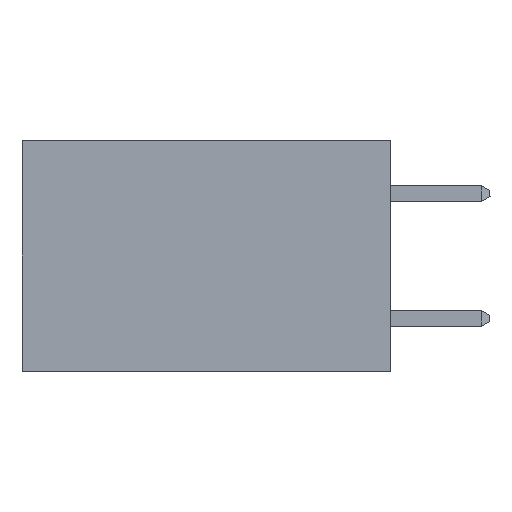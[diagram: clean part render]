
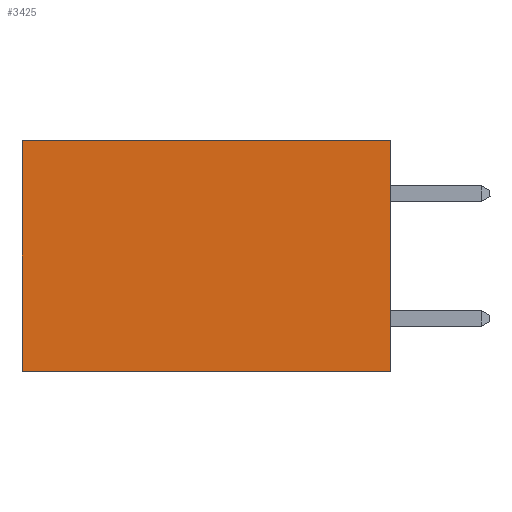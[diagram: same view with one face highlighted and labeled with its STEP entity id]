
A CAD part, left-side view. The second image highlights one B-rep face of the part: STEP entity #3425.
In plain terms, the highlighted planar face has unit normal (-1, 0, 0).
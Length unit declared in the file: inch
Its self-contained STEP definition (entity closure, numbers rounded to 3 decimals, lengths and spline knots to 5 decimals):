
#262 = VERTEX_POINT ( 'NONE', #16569 ) ;
#470 = CARTESIAN_POINT ( 'NONE',  ( 0.277, 0., -0.37 ) ) ;
#642 = AXIS2_PLACEMENT_3D ( 'NONE', #14936, #14911, #14886 ) ;
#1304 = DIRECTION ( 'NONE',  ( 0., 0., -1. ) ) ;
#1326 = CARTESIAN_POINT ( 'NONE',  ( 0.277, 0.59, -0.37 ) ) ;
#2081 = ORIENTED_EDGE ( 'NONE', *, *, #13320, .F. ) ;
#2238 = LINE ( 'NONE', #1326, #9989 ) ;
#3425 = ADVANCED_FACE ( 'NONE', ( #10855 ), #14974, .F. ) ;
#3613 = CARTESIAN_POINT ( 'NONE',  ( 0.277, 0., -0.37 ) ) ;
#3627 = ORIENTED_EDGE ( 'NONE', *, *, #12966, .T. ) ;
#4514 = VERTEX_POINT ( 'NONE', #11446 ) ;
#4677 = CARTESIAN_POINT ( 'NONE',  ( 0.277, 0.59, -0.37 ) ) ;
#5781 = CARTESIAN_POINT ( 'NONE',  ( 0.277, 0.59, 0. ) ) ;
#6550 = ORIENTED_EDGE ( 'NONE', *, *, #13348, .F. ) ;
#6610 = VECTOR ( 'NONE', #12892, 39.37008 ) ;
#8470 = LINE ( 'NONE', #3613, #12515 ) ;
#9789 = DIRECTION ( 'NONE',  ( 0., 1., 0. ) ) ;
#9901 = EDGE_CURVE ( 'NONE', #15641, #18014, #2238, .T. ) ;
#9989 = VECTOR ( 'NONE', #1304, 39.37008 ) ;
#10051 = ORIENTED_EDGE ( 'NONE', *, *, #9901, .T. ) ;
#10855 = FACE_OUTER_BOUND ( 'NONE', #15904, .T. ) ;
#11375 = CARTESIAN_POINT ( 'NONE',  ( 0.277, 0., 0. ) ) ;
#11410 = DIRECTION ( 'NONE',  ( 0., 0., -1. ) ) ;
#11446 = CARTESIAN_POINT ( 'NONE',  ( 0.277, 0., 0. ) ) ;
#11557 = VECTOR ( 'NONE', #11410, 39.37008 ) ;
#12515 = VECTOR ( 'NONE', #9789, 39.37008 ) ;
#12892 = DIRECTION ( 'NONE',  ( 0., 1., 0. ) ) ;
#12966 = EDGE_CURVE ( 'NONE', #4514, #15641, #14695, .T. ) ;
#13320 = EDGE_CURVE ( 'NONE', #262, #18014, #8470, .T. ) ;
#13348 = EDGE_CURVE ( 'NONE', #4514, #262, #15626, .T. ) ;
#14695 = LINE ( 'NONE', #11375, #6610 ) ;
#14886 = DIRECTION ( 'NONE',  ( 0., 0., -1. ) ) ;
#14911 = DIRECTION ( 'NONE',  ( 1., 0., 0. ) ) ;
#14936 = CARTESIAN_POINT ( 'NONE',  ( 0.277, 0., -0.37 ) ) ;
#14974 = PLANE ( 'NONE',  #642 ) ;
#15626 = LINE ( 'NONE', #470, #11557 ) ;
#15641 = VERTEX_POINT ( 'NONE', #5781 ) ;
#15904 = EDGE_LOOP ( 'NONE', ( #10051, #2081, #6550, #3627 ) ) ;
#16569 = CARTESIAN_POINT ( 'NONE',  ( 0.277, 0., -0.37 ) ) ;
#18014 = VERTEX_POINT ( 'NONE', #4677 ) ;
